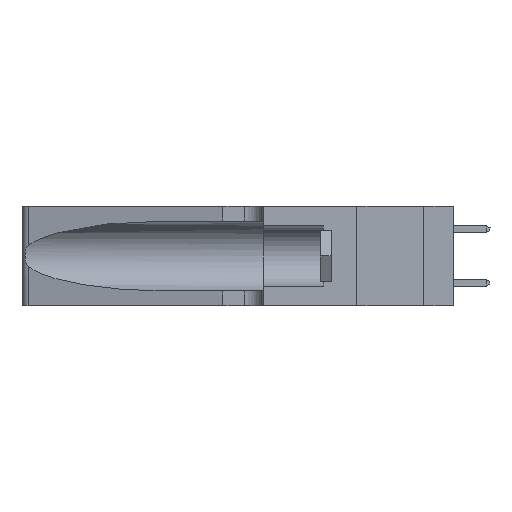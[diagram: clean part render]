
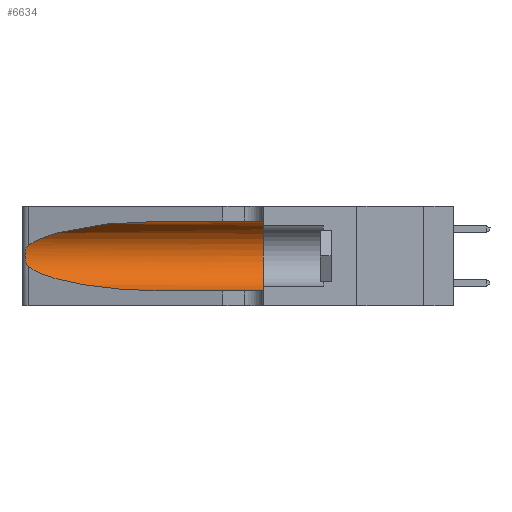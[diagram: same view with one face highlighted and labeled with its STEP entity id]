
A CAD part, left-side view. The second image highlights one B-rep face of the part: STEP entity #6634.
In plain terms, the highlighted cylindrical face has radius 3.308 mm (diameter 6.617 mm), a partial arc.
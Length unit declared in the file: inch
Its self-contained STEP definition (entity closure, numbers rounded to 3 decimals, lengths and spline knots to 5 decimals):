
#1441 = CARTESIAN_POINT ( 'NONE',  ( 0.1305, 0.35, 0.31525 ) ) ;
#2523 = CARTESIAN_POINT ( 'NONE',  ( 0.26017, 1.23833, 0.17102 ) ) ;
#2657 = CARTESIAN_POINT ( 'NONE',  ( 0.1305, 0.35, 0.05475 ) ) ;
#3938 = CARTESIAN_POINT ( 'NONE',  ( 0.1305, 0.72297, 0.31525 ) ) ;
#5933 = ORIENTED_EDGE ( 'NONE', *, *, #26347, .T. ) ;
#6060 = CYLINDRICAL_SURFACE ( 'NONE', #33894, 0.13025 ) ;
#6134 = EDGE_CURVE ( 'NONE', #39849, #30367, #43656, .T. ) ;
#6634 = ADVANCED_FACE ( 'NONE', ( #34146 ), #6060, .F. ) ;
#6758 = ORIENTED_EDGE ( 'NONE', *, *, #23153, .F. ) ;
#7099 = AXIS2_PLACEMENT_3D ( 'NONE', #7203, #13414, #13715 ) ;
#7203 = CARTESIAN_POINT ( 'NONE',  ( 0.1305, 0.35, 0.185 ) ) ;
#7531 = VERTEX_POINT ( 'NONE', #2657 ) ;
#8756 = CARTESIAN_POINT ( 'NONE',  ( 0.18966, 0.96281, 0.05475 ) ) ;
#10680 = LINE ( 'NONE', #35095, #24447 ) ;
#11733 = DIRECTION ( 'NONE',  ( 0., -1., 0. ) ) ;
#13414 = DIRECTION ( 'NONE',  ( 0., 1., 0. ) ) ;
#13582 = CIRCLE ( 'NONE', #7099, 0.13025 ) ;
#13715 = DIRECTION ( 'NONE',  ( 0., 0., 1. ) ) ;
#14138 = CARTESIAN_POINT ( 'NONE',  ( 0.2373, 1.15595, 0.28018 ) ) ;
#15700 = CARTESIAN_POINT ( 'NONE',  ( 0.25487, 1.22718, 0.14631 ) ) ;
#15949 = CARTESIAN_POINT ( 'NONE',  ( 0.25639, 1.23184, 0.21858 ) ) ;
#16658 = EDGE_CURVE ( 'NONE', #39849, #16773, #21333, .T. ) ;
#16773 = VERTEX_POINT ( 'NONE', #38534 ) ;
#17023 = CARTESIAN_POINT ( 'NONE',  ( 0.25487, 1.22718, 0.14631 ) ) ;
#17381 = VERTEX_POINT ( 'NONE', #17023 ) ;
#19182 = CARTESIAN_POINT ( 'NONE',  ( 0.25487, 1.22718, 0.22369 ) ) ;
#19326 = CARTESIAN_POINT ( 'NONE',  ( 0.25555, 1.22993, 0.14849 ) ) ;
#19350 = CARTESIAN_POINT ( 'NONE',  ( 0.2373, 1.15595, 0.08982 ) ) ;
#19937 = EDGE_LOOP ( 'NONE', ( #38260, #42462, #5933, #30413, #6758, #35824 ) ) ;
#20987 = CARTESIAN_POINT ( 'NONE',  ( 0.1305, 1.61858, 0.185 ) ) ;
#21333 =( BOUNDED_CURVE ( )  B_SPLINE_CURVE ( 3, ( #3938, #31276, #14138, #21344 ),
 .UNSPECIFIED., .F., .F. ) 
 B_SPLINE_CURVE_WITH_KNOTS ( ( 4, 4 ),
 ( 1.5708, 2.84003 ),
 .UNSPECIFIED. ) 
 CURVE ( )  GEOMETRIC_REPRESENTATION_ITEM ( )  RATIONAL_B_SPLINE_CURVE ( ( 1., 0.87, 0.87, 1. ) ) 
 REPRESENTATION_ITEM ( '' )  );
#21344 = CARTESIAN_POINT ( 'NONE',  ( 0.25487, 1.22718, 0.22369 ) ) ;
#22580 = CARTESIAN_POINT ( 'NONE',  ( 0.25555, 1.22994, 0.2215 ) ) ;
#23020 = CARTESIAN_POINT ( 'NONE',  ( 0.25787, 1.23484, 0.2124 ) ) ;
#23153 = EDGE_CURVE ( 'NONE', #30367, #7531, #13582, .T. ) ;
#24447 = VECTOR ( 'NONE', #11733, 39.37008 ) ;
#26018 = CARTESIAN_POINT ( 'NONE',  ( 0.25789, 1.23486, 0.15765 ) ) ;
#26163 = CARTESIAN_POINT ( 'NONE',  ( 0.25487, 1.22718, 0.14631 ) ) ;
#26347 = EDGE_CURVE ( 'NONE', #17381, #32939, #37484, .T. ) ;
#29389 = CARTESIAN_POINT ( 'NONE',  ( 0.25856, 1.23593, 0.16098 ) ) ;
#29672 = CARTESIAN_POINT ( 'NONE',  ( 0.26075, 1.23896, 0.178 ) ) ;
#30367 = VERTEX_POINT ( 'NONE', #1441 ) ;
#30413 = ORIENTED_EDGE ( 'NONE', *, *, #41867, .T. ) ;
#31276 = CARTESIAN_POINT ( 'NONE',  ( 0.18966, 0.96281, 0.31525 ) ) ;
#32939 = VERTEX_POINT ( 'NONE', #41873 ) ;
#33438 = B_SPLINE_CURVE_WITH_KNOTS ( 'NONE', 3,
 ( #19182, #22580, #15949, #23020, #39624, #43134, #36224, #29672, #2523, #29389, #26018, #39758, #19326, #26163 ),
 .UNSPECIFIED., .F., .F.,
 ( 4, 2, 2, 2, 2, 2, 4 ),
 ( 0., 0.00027, 0.00053, 0.00107, 0.0016, 0.00187, 0.00214 ),
 .UNSPECIFIED. ) ;
#33894 = AXIS2_PLACEMENT_3D ( 'NONE', #20987, #38777, #42170 ) ;
#34146 = FACE_OUTER_BOUND ( 'NONE', #19937, .T. ) ;
#34803 = EDGE_CURVE ( 'NONE', #16773, #17381, #33438, .T. ) ;
#35095 = CARTESIAN_POINT ( 'NONE',  ( 0.1305, 1.61858, 0.05475 ) ) ;
#35824 = ORIENTED_EDGE ( 'NONE', *, *, #6134, .F. ) ;
#36224 = CARTESIAN_POINT ( 'NONE',  ( 0.26075, 1.23896, 0.19203 ) ) ;
#37484 =( BOUNDED_CURVE ( )  B_SPLINE_CURVE ( 3, ( #15700, #19350, #8756, #43023 ),
 .UNSPECIFIED., .F., .T. ) 
 B_SPLINE_CURVE_WITH_KNOTS ( ( 4, 4 ),
 ( 3.44316, 4.71239 ),
 .UNSPECIFIED. ) 
 CURVE ( )  GEOMETRIC_REPRESENTATION_ITEM ( )  RATIONAL_B_SPLINE_CURVE ( ( 1., 0.87, 0.87, 1. ) ) 
 REPRESENTATION_ITEM ( '' )  );
#38260 = ORIENTED_EDGE ( 'NONE', *, *, #16658, .T. ) ;
#38534 = CARTESIAN_POINT ( 'NONE',  ( 0.25487, 1.22718, 0.22369 ) ) ;
#38777 = DIRECTION ( 'NONE',  ( 0., -1., 0. ) ) ;
#38997 = DIRECTION ( 'NONE',  ( 0., -1., 0. ) ) ;
#39624 = CARTESIAN_POINT ( 'NONE',  ( 0.25854, 1.2359, 0.20912 ) ) ;
#39758 = CARTESIAN_POINT ( 'NONE',  ( 0.25639, 1.23186, 0.15144 ) ) ;
#39849 = VERTEX_POINT ( 'NONE', #42202 ) ;
#40501 = VECTOR ( 'NONE', #38997, 39.37008 ) ;
#41867 = EDGE_CURVE ( 'NONE', #32939, #7531, #10680, .T. ) ;
#41873 = CARTESIAN_POINT ( 'NONE',  ( 0.1305, 0.72297, 0.05475 ) ) ;
#42170 = DIRECTION ( 'NONE',  ( 0., 0., -1. ) ) ;
#42202 = CARTESIAN_POINT ( 'NONE',  ( 0.1305, 0.72297, 0.31525 ) ) ;
#42205 = CARTESIAN_POINT ( 'NONE',  ( 0.1305, 1.61858, 0.31525 ) ) ;
#42462 = ORIENTED_EDGE ( 'NONE', *, *, #34803, .T. ) ;
#43023 = CARTESIAN_POINT ( 'NONE',  ( 0.1305, 0.72297, 0.05475 ) ) ;
#43134 = CARTESIAN_POINT ( 'NONE',  ( 0.26018, 1.23835, 0.19895 ) ) ;
#43656 = LINE ( 'NONE', #42205, #40501 ) ;
